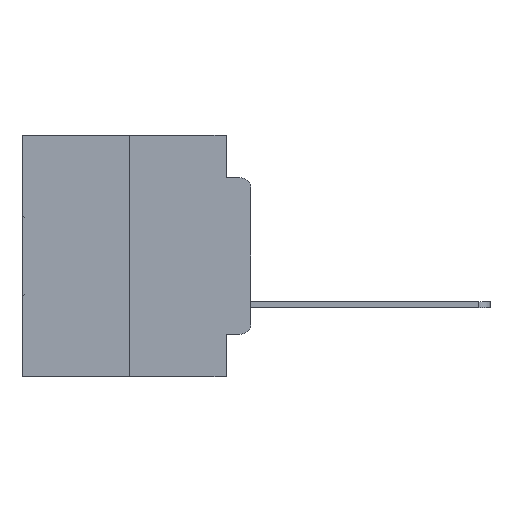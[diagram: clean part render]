
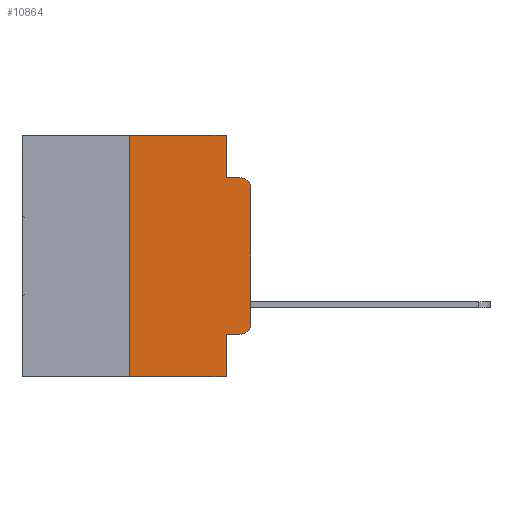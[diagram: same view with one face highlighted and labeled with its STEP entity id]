
A CAD part, left-side view. The second image highlights one B-rep face of the part: STEP entity #10864.
In plain terms, the highlighted planar face has unit normal (-1, 0, 0).
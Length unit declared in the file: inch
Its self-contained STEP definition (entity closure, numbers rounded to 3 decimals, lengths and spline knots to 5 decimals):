
#101 = CARTESIAN_POINT ( 'NONE',  ( 0., 0.473, 0. ) ) ;
#211 = CARTESIAN_POINT ( 'NONE',  ( 0., 0.051, 0. ) ) ;
#262 = DIRECTION ( 'NONE',  ( 0., 0., -1. ) ) ;
#302 = DIRECTION ( 'NONE',  ( 1., 0., 0. ) ) ;
#690 = FACE_OUTER_BOUND ( 'NONE', #5173, .T. ) ;
#1023 = VECTOR ( 'NONE', #12919, 39.37008 ) ;
#2061 = ORIENTED_EDGE ( 'NONE', *, *, #12762, .F. ) ;
#2178 = ORIENTED_EDGE ( 'NONE', *, *, #4159, .T. ) ;
#2486 = VERTEX_POINT ( 'NONE', #18866 ) ;
#4159 = EDGE_CURVE ( 'NONE', #9042, #15802, #26827, .T. ) ;
#4609 = CARTESIAN_POINT ( 'NONE',  ( 0., 0.051, -0.5 ) ) ;
#5043 = ORIENTED_EDGE ( 'NONE', *, *, #18294, .F. ) ;
#5173 = EDGE_LOOP ( 'NONE', ( #5458, #29124, #5043, #27231, #2061, #15416, #25332, #17437, #15450, #2178 ) ) ;
#5458 = ORIENTED_EDGE ( 'NONE', *, *, #23374, .T. ) ;
#5692 = CARTESIAN_POINT ( 'NONE',  ( 0., 0.051, 0. ) ) ;
#5694 = LINE ( 'NONE', #23753, #18784 ) ;
#5887 = VECTOR ( 'NONE', #20164, 39.37008 ) ;
#6012 = EDGE_CURVE ( 'NONE', #2486, #9042, #7616, .T. ) ;
#6192 = CARTESIAN_POINT ( 'NONE',  ( 0., 0.02, -0.0885 ) ) ;
#6617 = CARTESIAN_POINT ( 'NONE',  ( 0., 0.051, -0.0885 ) ) ;
#7616 = LINE ( 'NONE', #17504, #5887 ) ;
#7862 = EDGE_CURVE ( 'NONE', #2486, #30532, #31629, .T. ) ;
#9042 = VERTEX_POINT ( 'NONE', #25515 ) ;
#9119 = LINE ( 'NONE', #25536, #1023 ) ;
#9670 = EDGE_CURVE ( 'NONE', #21084, #30281, #32532, .T. ) ;
#10294 = VERTEX_POINT ( 'NONE', #20354 ) ;
#10483 = VERTEX_POINT ( 'NONE', #211 ) ;
#10864 = ADVANCED_FACE ( 'NONE', ( #690 ), #31171, .F. ) ;
#11226 = VECTOR ( 'NONE', #22082, 39.37008 ) ;
#11279 = LINE ( 'NONE', #101, #30552 ) ;
#11737 = VECTOR ( 'NONE', #30937, 39.37008 ) ;
#11931 = AXIS2_PLACEMENT_3D ( 'NONE', #27361, #12232, #29814 ) ;
#12232 = DIRECTION ( 'NONE',  ( -1., 0., 0. ) ) ;
#12656 = CARTESIAN_POINT ( 'NONE',  ( 0., 0., 0. ) ) ;
#12762 = EDGE_CURVE ( 'NONE', #30281, #10483, #11279, .T. ) ;
#12919 = DIRECTION ( 'NONE',  ( 0., 0., -1. ) ) ;
#13637 = LINE ( 'NONE', #12656, #26312 ) ;
#14529 = AXIS2_PLACEMENT_3D ( 'NONE', #30569, #15575, #33064 ) ;
#14860 = EDGE_CURVE ( 'NONE', #10483, #31862, #9119, .T. ) ;
#15214 = DIRECTION ( 'NONE',  ( 0., 0., 1. ) ) ;
#15416 = ORIENTED_EDGE ( 'NONE', *, *, #9670, .F. ) ;
#15450 = ORIENTED_EDGE ( 'NONE', *, *, #6012, .T. ) ;
#15575 = DIRECTION ( 'NONE',  ( -1., 0., 0. ) ) ;
#15802 = VERTEX_POINT ( 'NONE', #18764 ) ;
#15853 = CARTESIAN_POINT ( 'NONE',  ( 0., 0.25, 0. ) ) ;
#17437 = ORIENTED_EDGE ( 'NONE', *, *, #7862, .F. ) ;
#17504 = CARTESIAN_POINT ( 'NONE',  ( 0., 0.051, -0.4115 ) ) ;
#18092 = CIRCLE ( 'NONE', #11931, 0.02 ) ;
#18294 = EDGE_CURVE ( 'NONE', #31862, #28206, #24740, .T. ) ;
#18725 = EDGE_CURVE ( 'NONE', #21084, #30532, #5694, .T. ) ;
#18763 = DIRECTION ( 'NONE',  ( 0., 0., -1. ) ) ;
#18764 = CARTESIAN_POINT ( 'NONE',  ( 0., 0., -0.3915 ) ) ;
#18784 = VECTOR ( 'NONE', #26242, 39.37008 ) ;
#18866 = CARTESIAN_POINT ( 'NONE',  ( 0., 0.051, -0.4115 ) ) ;
#20164 = DIRECTION ( 'NONE',  ( 0., -1., 0. ) ) ;
#20354 = CARTESIAN_POINT ( 'NONE',  ( 0., 0., -0.1085 ) ) ;
#21084 = VERTEX_POINT ( 'NONE', #32097 ) ;
#21656 = EDGE_CURVE ( 'NONE', #10294, #28206, #18092, .T. ) ;
#22082 = DIRECTION ( 'NONE',  ( 0., -1., 0. ) ) ;
#23374 = EDGE_CURVE ( 'NONE', #15802, #10294, #13637, .T. ) ;
#23667 = DIRECTION ( 'NONE',  ( 0., -1., 0. ) ) ;
#23753 = CARTESIAN_POINT ( 'NONE',  ( 0., 0.473, -0.5 ) ) ;
#24740 = LINE ( 'NONE', #6617, #11226 ) ;
#25332 = ORIENTED_EDGE ( 'NONE', *, *, #18725, .T. ) ;
#25515 = CARTESIAN_POINT ( 'NONE',  ( 0., 0.02, -0.4115 ) ) ;
#25536 = CARTESIAN_POINT ( 'NONE',  ( 0., 0.051, 0. ) ) ;
#26242 = DIRECTION ( 'NONE',  ( 0., -1., 0. ) ) ;
#26312 = VECTOR ( 'NONE', #15214, 39.37008 ) ;
#26789 = AXIS2_PLACEMENT_3D ( 'NONE', #31066, #302, #18763 ) ;
#26827 = CIRCLE ( 'NONE', #14529, 0.02 ) ;
#26977 = CARTESIAN_POINT ( 'NONE',  ( 0., 0.25, 0. ) ) ;
#27231 = ORIENTED_EDGE ( 'NONE', *, *, #14860, .F. ) ;
#27361 = CARTESIAN_POINT ( 'NONE',  ( 0., 0.02, -0.1085 ) ) ;
#28206 = VERTEX_POINT ( 'NONE', #6192 ) ;
#29124 = ORIENTED_EDGE ( 'NONE', *, *, #21656, .T. ) ;
#29814 = DIRECTION ( 'NONE',  ( 0., 0., -1. ) ) ;
#30281 = VERTEX_POINT ( 'NONE', #26977 ) ;
#30532 = VERTEX_POINT ( 'NONE', #4609 ) ;
#30552 = VECTOR ( 'NONE', #23667, 39.37008 ) ;
#30569 = CARTESIAN_POINT ( 'NONE',  ( 0., 0.02, -0.3915 ) ) ;
#30857 = VECTOR ( 'NONE', #262, 39.37008 ) ;
#30937 = DIRECTION ( 'NONE',  ( 0., 0., 1. ) ) ;
#31066 = CARTESIAN_POINT ( 'NONE',  ( 0., 0.473, 0. ) ) ;
#31171 = PLANE ( 'NONE',  #26789 ) ;
#31629 = LINE ( 'NONE', #5692, #30857 ) ;
#31862 = VERTEX_POINT ( 'NONE', #32464 ) ;
#32097 = CARTESIAN_POINT ( 'NONE',  ( 0., 0.25, -0.5 ) ) ;
#32464 = CARTESIAN_POINT ( 'NONE',  ( 0., 0.051, -0.0885 ) ) ;
#32532 = LINE ( 'NONE', #15853, #11737 ) ;
#33064 = DIRECTION ( 'NONE',  ( 0., 0., -1. ) ) ;
